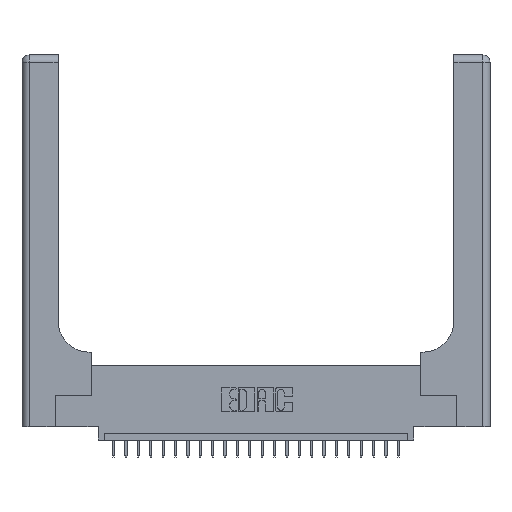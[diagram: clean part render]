
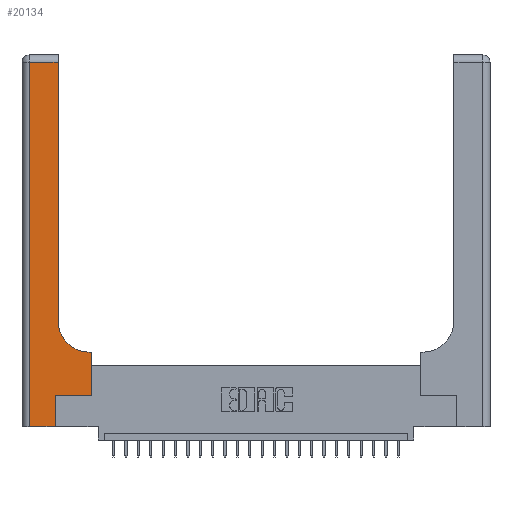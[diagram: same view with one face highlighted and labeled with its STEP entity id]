
A CAD part, top view. The second image highlights one B-rep face of the part: STEP entity #20134.
In plain terms, the highlighted planar face has unit normal (0, 0, 1).
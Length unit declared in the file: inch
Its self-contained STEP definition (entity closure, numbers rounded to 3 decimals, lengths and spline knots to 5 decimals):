
#1137 = AXIS2_PLACEMENT_3D ( 'NONE', #20843, #15208, #18735 ) ;
#1632 = ORIENTED_EDGE ( 'NONE', *, *, #7549, .T. ) ;
#1678 = CIRCLE ( 'NONE', #14640, 0.25 ) ;
#2053 = LINE ( 'NONE', #10298, #10745 ) ;
#2291 = EDGE_LOOP ( 'NONE', ( #7083, #24341, #18558, #17859, #12949, #2531, #19710, #1632, #16742 ) ) ;
#2531 = ORIENTED_EDGE ( 'NONE', *, *, #23993, .T. ) ;
#2731 = DIRECTION ( 'NONE',  ( -1., 0., 0. ) ) ;
#2956 = VECTOR ( 'NONE', #2731, 39.37008 ) ;
#3329 = CARTESIAN_POINT ( 'NONE',  ( 0.2915, 2.94, 0.37 ) ) ;
#3429 = DIRECTION ( 'NONE',  ( 1., 0., 0. ) ) ;
#3693 = LINE ( 'NONE', #21359, #9624 ) ;
#4144 = DIRECTION ( 'NONE',  ( 0., 1., 0. ) ) ;
#4565 = LINE ( 'NONE', #19286, #2956 ) ;
#4993 = LINE ( 'NONE', #12722, #22772 ) ;
#5166 = CARTESIAN_POINT ( 'NONE',  ( 0.269, 0.25, 0.37 ) ) ;
#5381 = CARTESIAN_POINT ( 'NONE',  ( 0.5415, 0.85, 0.37 ) ) ;
#5572 = VECTOR ( 'NONE', #6760, 39.37008 ) ;
#6234 = LINE ( 'NONE', #12136, #22470 ) ;
#6588 = DIRECTION ( 'NONE',  ( 0., 1., 0. ) ) ;
#6760 = DIRECTION ( 'NONE',  ( -1., 0., 0. ) ) ;
#6934 = VERTEX_POINT ( 'NONE', #9429 ) ;
#7083 = ORIENTED_EDGE ( 'NONE', *, *, #21328, .T. ) ;
#7100 = DIRECTION ( 'NONE',  ( 0., 0., -1. ) ) ;
#7427 = EDGE_CURVE ( 'NONE', #11314, #9121, #17754, .T. ) ;
#7549 = EDGE_CURVE ( 'NONE', #9121, #10003, #14617, .T. ) ;
#8475 = CARTESIAN_POINT ( 'NONE',  ( 0.2915, 0.6, 0.37 ) ) ;
#9121 = VERTEX_POINT ( 'NONE', #13307 ) ;
#9384 = EDGE_CURVE ( 'NONE', #20566, #16963, #4993, .T. ) ;
#9429 = CARTESIAN_POINT ( 'NONE',  ( 0.06, 0., 0.37 ) ) ;
#9624 = VECTOR ( 'NONE', #3429, 39.37008 ) ;
#10003 = VERTEX_POINT ( 'NONE', #21448 ) ;
#10298 = CARTESIAN_POINT ( 'NONE',  ( 0.06, 3., 0.37 ) ) ;
#10735 = VERTEX_POINT ( 'NONE', #3329 ) ;
#10745 = VECTOR ( 'NONE', #24425, 39.37008 ) ;
#11314 = VERTEX_POINT ( 'NONE', #20967 ) ;
#12136 = CARTESIAN_POINT ( 'NONE',  ( 0.2915, 3., 0.37 ) ) ;
#12722 = CARTESIAN_POINT ( 'NONE',  ( 0.269, 0., 0.37 ) ) ;
#12909 = EDGE_CURVE ( 'NONE', #19046, #6934, #2053, .T. ) ;
#12949 = ORIENTED_EDGE ( 'NONE', *, *, #9384, .T. ) ;
#13149 = LINE ( 'NONE', #5166, #18376 ) ;
#13307 = CARTESIAN_POINT ( 'NONE',  ( 0.5585, 0.6, 0.37 ) ) ;
#13368 = DIRECTION ( 'NONE',  ( 1., 0., 0. ) ) ;
#14189 = CARTESIAN_POINT ( 'NONE',  ( 0.269, 0., 0.37 ) ) ;
#14617 = LINE ( 'NONE', #8475, #5572 ) ;
#14640 = AXIS2_PLACEMENT_3D ( 'NONE', #5381, #7100, #13368 ) ;
#15083 = CARTESIAN_POINT ( 'NONE',  ( 0.2915, 0.85, 0.37 ) ) ;
#15208 = DIRECTION ( 'NONE',  ( 0., 0., -1. ) ) ;
#16742 = ORIENTED_EDGE ( 'NONE', *, *, #17088, .T. ) ;
#16963 = VERTEX_POINT ( 'NONE', #17158 ) ;
#17088 = EDGE_CURVE ( 'NONE', #10003, #24695, #1678, .T. ) ;
#17158 = CARTESIAN_POINT ( 'NONE',  ( 0.269, 0.25, 0.37 ) ) ;
#17754 = LINE ( 'NONE', #25745, #18092 ) ;
#17859 = ORIENTED_EDGE ( 'NONE', *, *, #24752, .T. ) ;
#17890 = DIRECTION ( 'NONE',  ( 0., 1., 0. ) ) ;
#18092 = VECTOR ( 'NONE', #17890, 39.37008 ) ;
#18376 = VECTOR ( 'NONE', #22961, 39.37008 ) ;
#18558 = ORIENTED_EDGE ( 'NONE', *, *, #12909, .T. ) ;
#18735 = DIRECTION ( 'NONE',  ( -1., 0., 0. ) ) ;
#19046 = VERTEX_POINT ( 'NONE', #25897 ) ;
#19286 = CARTESIAN_POINT ( 'NONE',  ( 0., 2.94, 0.37 ) ) ;
#19710 = ORIENTED_EDGE ( 'NONE', *, *, #7427, .T. ) ;
#20134 = ADVANCED_FACE ( 'NONE', ( #24640 ), #24765, .F. ) ;
#20566 = VERTEX_POINT ( 'NONE', #14189 ) ;
#20843 = CARTESIAN_POINT ( 'NONE',  ( 0., 3., 0.37 ) ) ;
#20967 = CARTESIAN_POINT ( 'NONE',  ( 0.5585, 0.25, 0.37 ) ) ;
#21328 = EDGE_CURVE ( 'NONE', #24695, #10735, #6234, .T. ) ;
#21359 = CARTESIAN_POINT ( 'NONE',  ( 0., 0., 0.37 ) ) ;
#21448 = CARTESIAN_POINT ( 'NONE',  ( 0.5415, 0.6, 0.37 ) ) ;
#22470 = VECTOR ( 'NONE', #4144, 39.37008 ) ;
#22772 = VECTOR ( 'NONE', #6588, 39.37008 ) ;
#22961 = DIRECTION ( 'NONE',  ( 1., 0., 0. ) ) ;
#23993 = EDGE_CURVE ( 'NONE', #16963, #11314, #13149, .T. ) ;
#24341 = ORIENTED_EDGE ( 'NONE', *, *, #25446, .T. ) ;
#24425 = DIRECTION ( 'NONE',  ( 0., -1., 0. ) ) ;
#24640 = FACE_OUTER_BOUND ( 'NONE', #2291, .T. ) ;
#24695 = VERTEX_POINT ( 'NONE', #15083 ) ;
#24752 = EDGE_CURVE ( 'NONE', #6934, #20566, #3693, .T. ) ;
#24765 = PLANE ( 'NONE',  #1137 ) ;
#25446 = EDGE_CURVE ( 'NONE', #10735, #19046, #4565, .T. ) ;
#25745 = CARTESIAN_POINT ( 'NONE',  ( 0.5585, 0.25, 0.37 ) ) ;
#25897 = CARTESIAN_POINT ( 'NONE',  ( 0.06, 2.94, 0.37 ) ) ;
